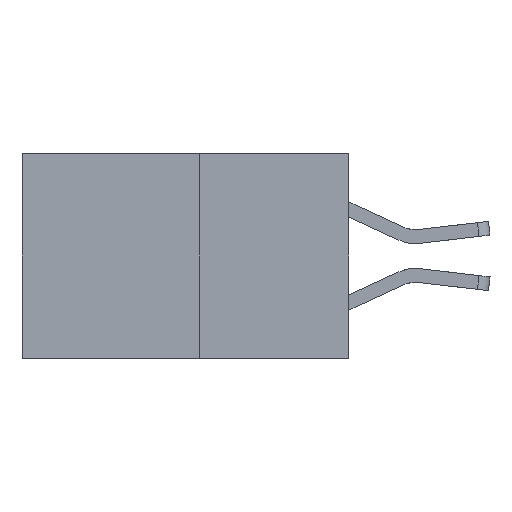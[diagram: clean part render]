
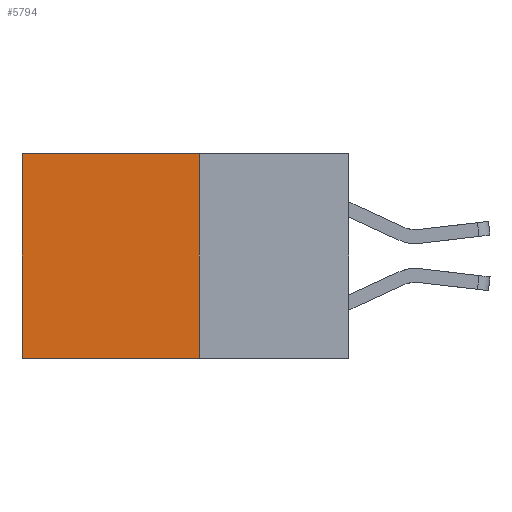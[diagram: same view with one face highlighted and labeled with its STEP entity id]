
A CAD part, left-side view. The second image highlights one B-rep face of the part: STEP entity #5794.
In plain terms, the highlighted planar face has unit normal (-1, 0, 0).
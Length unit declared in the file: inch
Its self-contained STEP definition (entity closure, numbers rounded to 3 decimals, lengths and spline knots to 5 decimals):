
#269 = LINE ( 'NONE', #6313, #8604 ) ;
#958 = CARTESIAN_POINT ( 'NONE',  ( 0.277, 0.27, 0. ) ) ;
#1304 = AXIS2_PLACEMENT_3D ( 'NONE', #7572, #7457, #7406 ) ;
#1640 = CARTESIAN_POINT ( 'NONE',  ( 0.277, 0.59, -0.37 ) ) ;
#1943 = VECTOR ( 'NONE', #9167, 39.37008 ) ;
#2771 = ORIENTED_EDGE ( 'NONE', *, *, #2924, .T. ) ;
#2795 = LINE ( 'NONE', #958, #8774 ) ;
#2924 = EDGE_CURVE ( 'NONE', #6167, #8171, #2795, .T. ) ;
#3904 = EDGE_LOOP ( 'NONE', ( #6709, #7515, #5476, #2771 ) ) ;
#4176 = CARTESIAN_POINT ( 'NONE',  ( 0.277, 0.27, 0. ) ) ;
#5203 = CARTESIAN_POINT ( 'NONE',  ( 0.277, 0.27, -0.37 ) ) ;
#5382 = FACE_OUTER_BOUND ( 'NONE', #3904, .T. ) ;
#5476 = ORIENTED_EDGE ( 'NONE', *, *, #10116, .F. ) ;
#5622 = CARTESIAN_POINT ( 'NONE',  ( 0.277, 0.27, -0.37 ) ) ;
#5794 = ADVANCED_FACE ( 'NONE', ( #5382 ), #7584, .F. ) ;
#5878 = EDGE_CURVE ( 'NONE', #5907, #7241, #269, .T. ) ;
#5907 = VERTEX_POINT ( 'NONE', #5622 ) ;
#6167 = VERTEX_POINT ( 'NONE', #4176 ) ;
#6249 = DIRECTION ( 'NONE',  ( 0., 1., 0. ) ) ;
#6313 = CARTESIAN_POINT ( 'NONE',  ( 0.277, 0.27, -0.37 ) ) ;
#6569 = DIRECTION ( 'NONE',  ( 0., 1., 0. ) ) ;
#6709 = ORIENTED_EDGE ( 'NONE', *, *, #9881, .T. ) ;
#7241 = VERTEX_POINT ( 'NONE', #1640 ) ;
#7406 = DIRECTION ( 'NONE',  ( 0., 0., -1. ) ) ;
#7457 = DIRECTION ( 'NONE',  ( 1., 0., 0. ) ) ;
#7515 = ORIENTED_EDGE ( 'NONE', *, *, #5878, .F. ) ;
#7572 = CARTESIAN_POINT ( 'NONE',  ( 0.277, 0.27, -0.37 ) ) ;
#7584 = PLANE ( 'NONE',  #1304 ) ;
#8149 = LINE ( 'NONE', #10509, #10206 ) ;
#8171 = VERTEX_POINT ( 'NONE', #8608 ) ;
#8196 = DIRECTION ( 'NONE',  ( 0., 0., -1. ) ) ;
#8498 = LINE ( 'NONE', #5203, #1943 ) ;
#8604 = VECTOR ( 'NONE', #6249, 39.37008 ) ;
#8608 = CARTESIAN_POINT ( 'NONE',  ( 0.277, 0.59, 0. ) ) ;
#8774 = VECTOR ( 'NONE', #6569, 39.37008 ) ;
#9167 = DIRECTION ( 'NONE',  ( 0., 0., -1. ) ) ;
#9881 = EDGE_CURVE ( 'NONE', #8171, #7241, #8149, .T. ) ;
#10116 = EDGE_CURVE ( 'NONE', #6167, #5907, #8498, .T. ) ;
#10206 = VECTOR ( 'NONE', #8196, 39.37008 ) ;
#10509 = CARTESIAN_POINT ( 'NONE',  ( 0.277, 0.59, -0.37 ) ) ;
